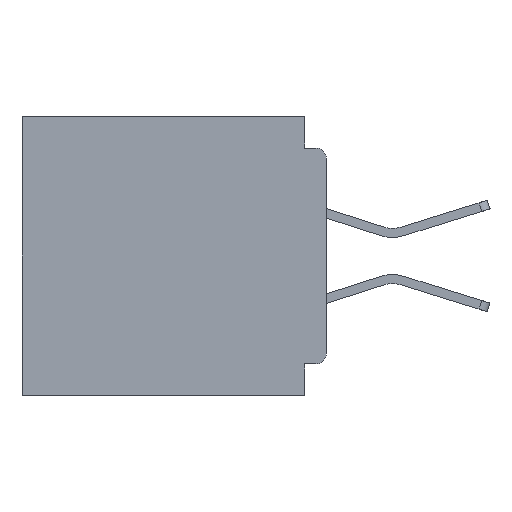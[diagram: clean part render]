
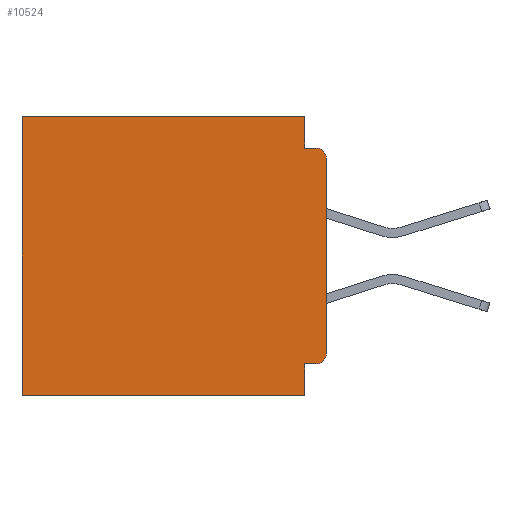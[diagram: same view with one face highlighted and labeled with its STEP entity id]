
A CAD part, left-side view. The second image highlights one B-rep face of the part: STEP entity #10524.
In plain terms, the highlighted planar face has unit normal (-1, 0, 0).
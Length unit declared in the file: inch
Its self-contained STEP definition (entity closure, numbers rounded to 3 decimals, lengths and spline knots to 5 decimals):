
#37 = DIRECTION ( 'NONE',  ( 0., 0., -1. ) ) ;
#1243 = CARTESIAN_POINT ( 'NONE',  ( 0.3, 0.031, 0. ) ) ;
#1356 = EDGE_LOOP ( 'NONE', ( #7757, #5847, #41906, #19484, #9734, #21558, #7433, #7730, #48125, #41367 ) ) ;
#1593 = CARTESIAN_POINT ( 'NONE',  ( 0.3, 0., -0.34 ) ) ;
#2561 = EDGE_CURVE ( 'NONE', #48093, #59586, #29252, .T. ) ;
#3581 = AXIS2_PLACEMENT_3D ( 'NONE', #53215, #24910, #57981 ) ;
#4023 = VECTOR ( 'NONE', #56524, 39.37008 ) ;
#4475 = CARTESIAN_POINT ( 'NONE',  ( 0.3, 0.015, -0.06 ) ) ;
#5497 = LINE ( 'NONE', #61259, #4023 ) ;
#5847 = ORIENTED_EDGE ( 'NONE', *, *, #22404, .T. ) ;
#7433 = ORIENTED_EDGE ( 'NONE', *, *, #34189, .F. ) ;
#7730 = ORIENTED_EDGE ( 'NONE', *, *, #18106, .F. ) ;
#7757 = ORIENTED_EDGE ( 'NONE', *, *, #2561, .F. ) ;
#8624 = CARTESIAN_POINT ( 'NONE',  ( 0.3, 0.031, 0. ) ) ;
#8714 = VERTEX_POINT ( 'NONE', #8624 ) ;
#9049 = PLANE ( 'NONE',  #38654 ) ;
#9266 = DIRECTION ( 'NONE',  ( 0., 0., -1. ) ) ;
#9734 = ORIENTED_EDGE ( 'NONE', *, *, #45567, .T. ) ;
#10524 = ADVANCED_FACE ( 'NONE', ( #60576 ), #9049, .F. ) ;
#12822 = DIRECTION ( 'NONE',  ( 0., -1., 0. ) ) ;
#13843 = DIRECTION ( 'NONE',  ( 0., 0., -1. ) ) ;
#14401 = VERTEX_POINT ( 'NONE', #30385 ) ;
#14981 = CARTESIAN_POINT ( 'NONE',  ( 0.3, 0.437, -0.4 ) ) ;
#15340 = DIRECTION ( 'NONE',  ( 0., 1., 0. ) ) ;
#16453 = VERTEX_POINT ( 'NONE', #51791 ) ;
#16593 = CARTESIAN_POINT ( 'NONE',  ( 0.3, 0.031, -0.045 ) ) ;
#16681 = VECTOR ( 'NONE', #37, 39.37008 ) ;
#18096 = CARTESIAN_POINT ( 'NONE',  ( 0.3, 0., -0.06 ) ) ;
#18106 = EDGE_CURVE ( 'NONE', #16453, #55467, #49218, .T. ) ;
#18527 = EDGE_CURVE ( 'NONE', #26542, #59586, #20885, .T. ) ;
#19484 = ORIENTED_EDGE ( 'NONE', *, *, #58884, .F. ) ;
#20885 = CIRCLE ( 'NONE', #3581, 0.015 ) ;
#21558 = ORIENTED_EDGE ( 'NONE', *, *, #43222, .T. ) ;
#21854 = VECTOR ( 'NONE', #15340, 39.37008 ) ;
#22404 = EDGE_CURVE ( 'NONE', #48093, #14401, #50748, .T. ) ;
#22978 = VECTOR ( 'NONE', #60132, 39.37008 ) ;
#24455 = LINE ( 'NONE', #55367, #22978 ) ;
#24460 = CARTESIAN_POINT ( 'NONE',  ( 0.3, 0., -0.355 ) ) ;
#24910 = DIRECTION ( 'NONE',  ( -1., 0., 0. ) ) ;
#25177 = DIRECTION ( 'NONE',  ( 0., 0., -1. ) ) ;
#26542 = VERTEX_POINT ( 'NONE', #61421 ) ;
#27032 = VECTOR ( 'NONE', #36095, 39.37008 ) ;
#27919 = DIRECTION ( 'NONE',  ( 1., 0., 0. ) ) ;
#27965 = LINE ( 'NONE', #60020, #39043 ) ;
#28207 = VERTEX_POINT ( 'NONE', #16593 ) ;
#29162 = DIRECTION ( 'NONE',  ( 0., 1., 0. ) ) ;
#29252 = LINE ( 'NONE', #57141, #16681 ) ;
#30385 = CARTESIAN_POINT ( 'NONE',  ( 0.3, 0.015, -0.045 ) ) ;
#32037 = CARTESIAN_POINT ( 'NONE',  ( 0.3, 0.437, 0. ) ) ;
#32916 = VECTOR ( 'NONE', #25177, 39.37008 ) ;
#34148 = CARTESIAN_POINT ( 'NONE',  ( 0.3, 0., -0.4 ) ) ;
#34189 = EDGE_CURVE ( 'NONE', #55467, #57654, #59579, .T. ) ;
#36095 = DIRECTION ( 'NONE',  ( 0., 0., -1. ) ) ;
#37424 = CARTESIAN_POINT ( 'NONE',  ( 0.3, 0., -0.4 ) ) ;
#37638 = DIRECTION ( 'NONE',  ( -1., 0., 0. ) ) ;
#37939 = EDGE_CURVE ( 'NONE', #28207, #14401, #27965, .T. ) ;
#38654 = AXIS2_PLACEMENT_3D ( 'NONE', #37424, #27919, #13843 ) ;
#39004 = CARTESIAN_POINT ( 'NONE',  ( 0.3, 0.031, -0.4 ) ) ;
#39043 = VECTOR ( 'NONE', #12822, 39.37008 ) ;
#41367 = ORIENTED_EDGE ( 'NONE', *, *, #18527, .T. ) ;
#41906 = ORIENTED_EDGE ( 'NONE', *, *, #37939, .F. ) ;
#43222 = EDGE_CURVE ( 'NONE', #53196, #57654, #5497, .T. ) ;
#45432 = LINE ( 'NONE', #1243, #32916 ) ;
#45567 = EDGE_CURVE ( 'NONE', #8714, #53196, #24455, .T. ) ;
#45890 = VECTOR ( 'NONE', #29162, 39.37008 ) ;
#48093 = VERTEX_POINT ( 'NONE', #18096 ) ;
#48125 = ORIENTED_EDGE ( 'NONE', *, *, #54735, .F. ) ;
#49218 = LINE ( 'NONE', #59698, #27032 ) ;
#49758 = AXIS2_PLACEMENT_3D ( 'NONE', #4475, #37638, #9266 ) ;
#50748 = CIRCLE ( 'NONE', #49758, 0.015 ) ;
#51791 = CARTESIAN_POINT ( 'NONE',  ( 0.3, 0.031, -0.355 ) ) ;
#53196 = VERTEX_POINT ( 'NONE', #32037 ) ;
#53215 = CARTESIAN_POINT ( 'NONE',  ( 0.3, 0.015, -0.34 ) ) ;
#54735 = EDGE_CURVE ( 'NONE', #26542, #16453, #60011, .T. ) ;
#55367 = CARTESIAN_POINT ( 'NONE',  ( 0.3, 0., 0. ) ) ;
#55467 = VERTEX_POINT ( 'NONE', #39004 ) ;
#56524 = DIRECTION ( 'NONE',  ( 0., 0., -1. ) ) ;
#57141 = CARTESIAN_POINT ( 'NONE',  ( 0.3, 0., -0.4 ) ) ;
#57654 = VERTEX_POINT ( 'NONE', #14981 ) ;
#57981 = DIRECTION ( 'NONE',  ( 0., 0., -1. ) ) ;
#58884 = EDGE_CURVE ( 'NONE', #8714, #28207, #45432, .T. ) ;
#59579 = LINE ( 'NONE', #34148, #21854 ) ;
#59586 = VERTEX_POINT ( 'NONE', #1593 ) ;
#59698 = CARTESIAN_POINT ( 'NONE',  ( 0.3, 0.031, -0.4 ) ) ;
#60011 = LINE ( 'NONE', #24460, #45890 ) ;
#60020 = CARTESIAN_POINT ( 'NONE',  ( 0.3, 0., -0.045 ) ) ;
#60132 = DIRECTION ( 'NONE',  ( 0., 1., 0. ) ) ;
#60576 = FACE_OUTER_BOUND ( 'NONE', #1356, .T. ) ;
#61259 = CARTESIAN_POINT ( 'NONE',  ( 0.3, 0.437, -0.4 ) ) ;
#61421 = CARTESIAN_POINT ( 'NONE',  ( 0.3, 0.015, -0.355 ) ) ;
